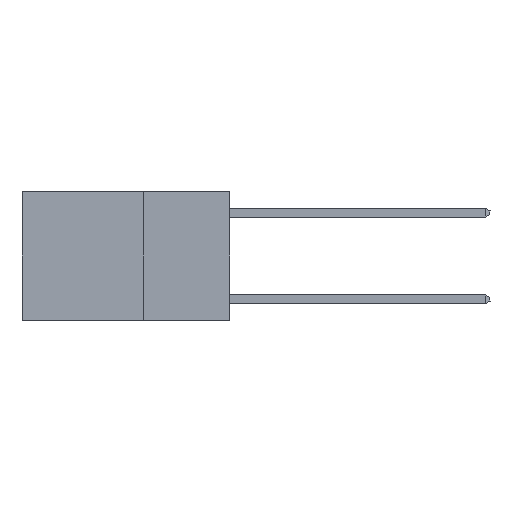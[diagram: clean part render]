
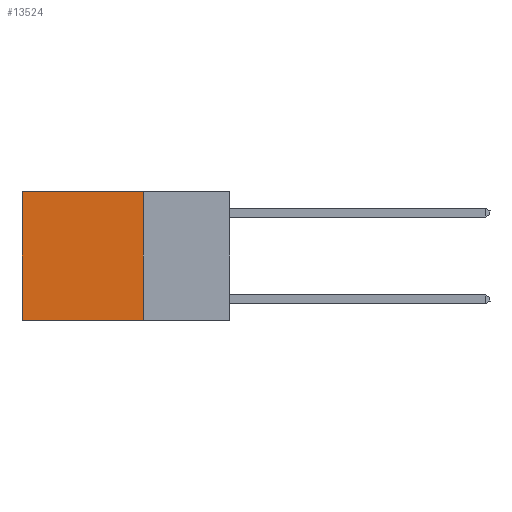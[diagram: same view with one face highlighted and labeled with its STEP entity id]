
A CAD part, left-side view. The second image highlights one B-rep face of the part: STEP entity #13524.
In plain terms, the highlighted planar face has unit normal (-1, 0, 0).
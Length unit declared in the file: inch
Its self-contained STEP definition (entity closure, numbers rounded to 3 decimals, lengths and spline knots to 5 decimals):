
#1612 = PLANE ( 'NONE',  #9027 ) ;
#1910 = CARTESIAN_POINT ( 'NONE',  ( 0.2625, 0.25, 0. ) ) ;
#2046 = EDGE_CURVE ( 'NONE', #8380, #9997, #5419, .T. ) ;
#2164 = LINE ( 'NONE', #17219, #6685 ) ;
#3122 = CARTESIAN_POINT ( 'NONE',  ( 0.2625, 0.25, -0.37 ) ) ;
#3185 = VERTEX_POINT ( 'NONE', #7553 ) ;
#3725 = LINE ( 'NONE', #9978, #18809 ) ;
#4983 = ORIENTED_EDGE ( 'NONE', *, *, #12981, .F. ) ;
#5419 = LINE ( 'NONE', #5609, #7901 ) ;
#5609 = CARTESIAN_POINT ( 'NONE',  ( 0.2625, 0.25, 0. ) ) ;
#6685 = VECTOR ( 'NONE', #10040, 39.37008 ) ;
#7482 = EDGE_CURVE ( 'NONE', #9997, #3185, #2164, .T. ) ;
#7553 = CARTESIAN_POINT ( 'NONE',  ( 0.2625, 0.6, -0.37 ) ) ;
#7779 = DIRECTION ( 'NONE',  ( 1., 0., 0. ) ) ;
#7901 = VECTOR ( 'NONE', #8853, 39.37008 ) ;
#8380 = VERTEX_POINT ( 'NONE', #10492 ) ;
#8386 = ORIENTED_EDGE ( 'NONE', *, *, #2046, .T. ) ;
#8853 = DIRECTION ( 'NONE',  ( 0., 1., 0. ) ) ;
#9027 = AXIS2_PLACEMENT_3D ( 'NONE', #1910, #7779, #12415 ) ;
#9655 = ORIENTED_EDGE ( 'NONE', *, *, #13611, .F. ) ;
#9978 = CARTESIAN_POINT ( 'NONE',  ( 0.2625, 0.25, -0.37 ) ) ;
#9997 = VERTEX_POINT ( 'NONE', #19500 ) ;
#10040 = DIRECTION ( 'NONE',  ( 0., 0., -1. ) ) ;
#10492 = CARTESIAN_POINT ( 'NONE',  ( 0.2625, 0.25, 0. ) ) ;
#12415 = DIRECTION ( 'NONE',  ( 0., 0., -1. ) ) ;
#12764 = CARTESIAN_POINT ( 'NONE',  ( 0.2625, 0.25, 0. ) ) ;
#12869 = DIRECTION ( 'NONE',  ( 0., 0., -1. ) ) ;
#12981 = EDGE_CURVE ( 'NONE', #8380, #17031, #14072, .T. ) ;
#13524 = ADVANCED_FACE ( 'NONE', ( #15497 ), #1612, .F. ) ;
#13611 = EDGE_CURVE ( 'NONE', #17031, #3185, #3725, .T. ) ;
#14072 = LINE ( 'NONE', #12764, #16153 ) ;
#15497 = FACE_OUTER_BOUND ( 'NONE', #18443, .T. ) ;
#16153 = VECTOR ( 'NONE', #12869, 39.37008 ) ;
#16193 = DIRECTION ( 'NONE',  ( 0., 1., 0. ) ) ;
#17031 = VERTEX_POINT ( 'NONE', #3122 ) ;
#17219 = CARTESIAN_POINT ( 'NONE',  ( 0.2625, 0.6, 0. ) ) ;
#18059 = ORIENTED_EDGE ( 'NONE', *, *, #7482, .T. ) ;
#18443 = EDGE_LOOP ( 'NONE', ( #18059, #9655, #4983, #8386 ) ) ;
#18809 = VECTOR ( 'NONE', #16193, 39.37008 ) ;
#19500 = CARTESIAN_POINT ( 'NONE',  ( 0.2625, 0.6, 0. ) ) ;
